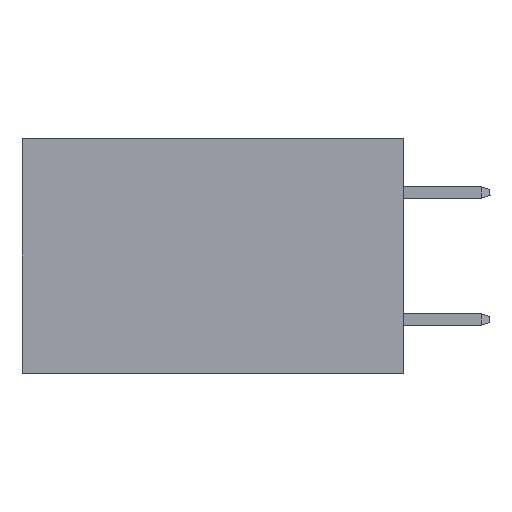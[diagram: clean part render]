
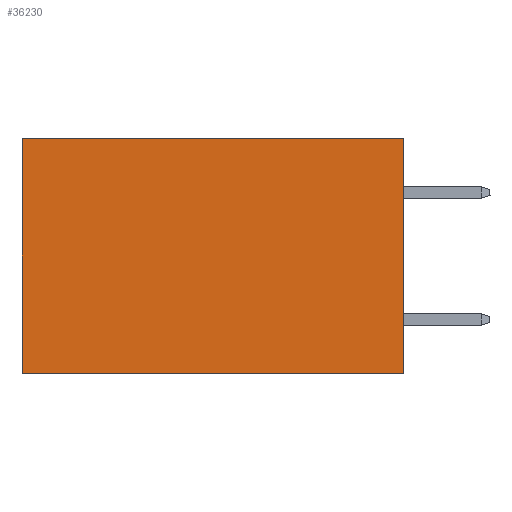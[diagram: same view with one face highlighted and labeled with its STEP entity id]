
A CAD part, left-side view. The second image highlights one B-rep face of the part: STEP entity #36230.
In plain terms, the highlighted planar face has unit normal (-1, 0, 0).
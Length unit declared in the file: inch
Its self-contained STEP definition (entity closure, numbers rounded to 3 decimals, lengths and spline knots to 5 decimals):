
#912 = DIRECTION ( 'NONE',  ( 0., 1., 0. ) ) ;
#1074 = VERTEX_POINT ( 'NONE', #5260 ) ;
#4996 = EDGE_LOOP ( 'NONE', ( #17653, #17323, #29097, #19319 ) ) ;
#5260 = CARTESIAN_POINT ( 'NONE',  ( 0.2875, 0.6, -0.37 ) ) ;
#6852 = CARTESIAN_POINT ( 'NONE',  ( 0.2875, 0.6, 0. ) ) ;
#11414 = AXIS2_PLACEMENT_3D ( 'NONE', #28257, #21880, #13157 ) ;
#12153 = CARTESIAN_POINT ( 'NONE',  ( 0.2875, 0., 0. ) ) ;
#13157 = DIRECTION ( 'NONE',  ( 0., 0., -1. ) ) ;
#15131 = DIRECTION ( 'NONE',  ( 0., 0., -1. ) ) ;
#15279 = FACE_OUTER_BOUND ( 'NONE', #4996, .T. ) ;
#17323 = ORIENTED_EDGE ( 'NONE', *, *, #39161, .F. ) ;
#17653 = ORIENTED_EDGE ( 'NONE', *, *, #40513, .T. ) ;
#19319 = ORIENTED_EDGE ( 'NONE', *, *, #25183, .T. ) ;
#20416 = VERTEX_POINT ( 'NONE', #32728 ) ;
#21505 = LINE ( 'NONE', #12153, #31094 ) ;
#21880 = DIRECTION ( 'NONE',  ( 1., 0., 0. ) ) ;
#23810 = DIRECTION ( 'NONE',  ( 0., 1., 0. ) ) ;
#24844 = VECTOR ( 'NONE', #23810, 39.37008 ) ;
#25183 = EDGE_CURVE ( 'NONE', #25885, #35905, #39561, .T. ) ;
#25885 = VERTEX_POINT ( 'NONE', #38353 ) ;
#26552 = CARTESIAN_POINT ( 'NONE',  ( 0.2875, 0., -0.37 ) ) ;
#27677 = EDGE_CURVE ( 'NONE', #25885, #20416, #21505, .T. ) ;
#28257 = CARTESIAN_POINT ( 'NONE',  ( 0.2875, 0., 0. ) ) ;
#28860 = LINE ( 'NONE', #30151, #31348 ) ;
#29097 = ORIENTED_EDGE ( 'NONE', *, *, #27677, .F. ) ;
#30151 = CARTESIAN_POINT ( 'NONE',  ( 0.2875, 0.6, 0. ) ) ;
#31094 = VECTOR ( 'NONE', #15131, 39.37008 ) ;
#31348 = VECTOR ( 'NONE', #36509, 39.37008 ) ;
#31470 = PLANE ( 'NONE',  #11414 ) ;
#32728 = CARTESIAN_POINT ( 'NONE',  ( 0.2875, 0., -0.37 ) ) ;
#33379 = LINE ( 'NONE', #26552, #37368 ) ;
#35905 = VERTEX_POINT ( 'NONE', #6852 ) ;
#36230 = ADVANCED_FACE ( 'NONE', ( #15279 ), #31470, .F. ) ;
#36509 = DIRECTION ( 'NONE',  ( 0., 0., -1. ) ) ;
#36996 = CARTESIAN_POINT ( 'NONE',  ( 0.2875, 0., 0. ) ) ;
#37368 = VECTOR ( 'NONE', #912, 39.37008 ) ;
#38353 = CARTESIAN_POINT ( 'NONE',  ( 0.2875, 0., 0. ) ) ;
#39161 = EDGE_CURVE ( 'NONE', #20416, #1074, #33379, .T. ) ;
#39561 = LINE ( 'NONE', #36996, #24844 ) ;
#40513 = EDGE_CURVE ( 'NONE', #35905, #1074, #28860, .T. ) ;
